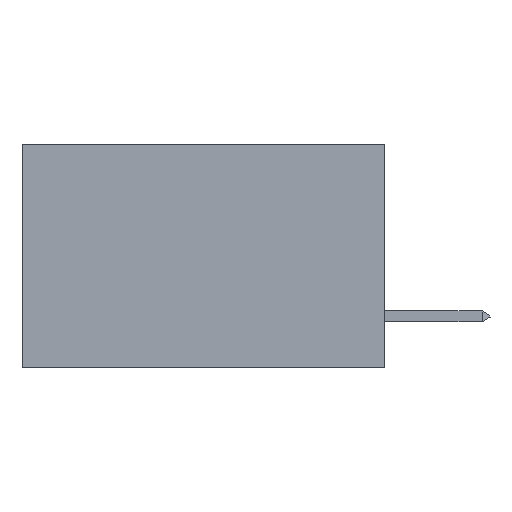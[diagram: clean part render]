
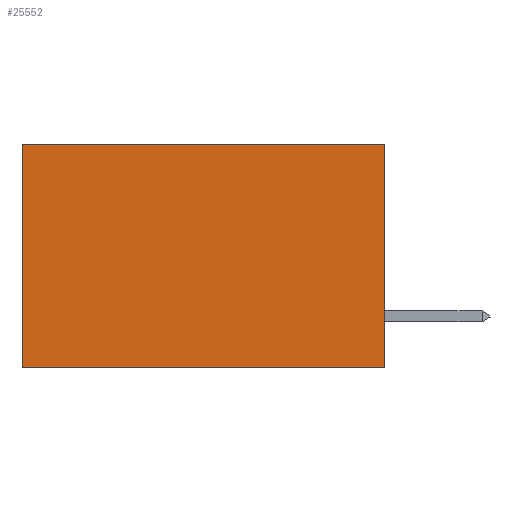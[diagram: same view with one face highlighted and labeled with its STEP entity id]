
A CAD part, left-side view. The second image highlights one B-rep face of the part: STEP entity #25552.
In plain terms, the highlighted planar face has unit normal (-1, 0, 0).
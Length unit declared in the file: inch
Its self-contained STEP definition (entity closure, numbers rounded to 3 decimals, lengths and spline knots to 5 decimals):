
#113 = EDGE_LOOP ( 'NONE', ( #18120, #8792, #2222, #19200 ) ) ;
#640 = DIRECTION ( 'NONE',  ( 0., 1., 0. ) ) ;
#1634 = VERTEX_POINT ( 'NONE', #12951 ) ;
#2222 = ORIENTED_EDGE ( 'NONE', *, *, #30428, .F. ) ;
#2575 = DIRECTION ( 'NONE',  ( 0., 0., -1. ) ) ;
#3344 = DIRECTION ( 'NONE',  ( 0., 0., -1. ) ) ;
#3620 = CARTESIAN_POINT ( 'NONE',  ( 0.2875, 0., -0.37 ) ) ;
#7477 = FACE_OUTER_BOUND ( 'NONE', #113, .T. ) ;
#8740 = LINE ( 'NONE', #19917, #25489 ) ;
#8792 = ORIENTED_EDGE ( 'NONE', *, *, #28315, .F. ) ;
#12466 = VERTEX_POINT ( 'NONE', #20766 ) ;
#12951 = CARTESIAN_POINT ( 'NONE',  ( 0.2875, 0., 0. ) ) ;
#13256 = VECTOR ( 'NONE', #23336, 39.37008 ) ;
#13271 = CARTESIAN_POINT ( 'NONE',  ( 0.2875, 0., 0. ) ) ;
#15188 = VECTOR ( 'NONE', #3344, 39.37008 ) ;
#17224 = DIRECTION ( 'NONE',  ( 0., 0., -1. ) ) ;
#18120 = ORIENTED_EDGE ( 'NONE', *, *, #25185, .T. ) ;
#18304 = CARTESIAN_POINT ( 'NONE',  ( 0.2875, 0.6, -0.37 ) ) ;
#18624 = PLANE ( 'NONE',  #26337 ) ;
#18912 = LINE ( 'NONE', #13271, #15188 ) ;
#19200 = ORIENTED_EDGE ( 'NONE', *, *, #26261, .T. ) ;
#19917 = CARTESIAN_POINT ( 'NONE',  ( 0.2875, 0.6, 0. ) ) ;
#20766 = CARTESIAN_POINT ( 'NONE',  ( 0.2875, 0., -0.37 ) ) ;
#23336 = DIRECTION ( 'NONE',  ( 0., 1., 0. ) ) ;
#23638 = CARTESIAN_POINT ( 'NONE',  ( 0.2875, 0., 0. ) ) ;
#23996 = VERTEX_POINT ( 'NONE', #31749 ) ;
#24476 = VECTOR ( 'NONE', #640, 39.37008 ) ;
#25185 = EDGE_CURVE ( 'NONE', #23996, #28552, #8740, .T. ) ;
#25489 = VECTOR ( 'NONE', #17224, 39.37008 ) ;
#25552 = ADVANCED_FACE ( 'NONE', ( #7477 ), #18624, .F. ) ;
#26261 = EDGE_CURVE ( 'NONE', #1634, #23996, #29100, .T. ) ;
#26337 = AXIS2_PLACEMENT_3D ( 'NONE', #23638, #34285, #2575 ) ;
#28315 = EDGE_CURVE ( 'NONE', #12466, #28552, #29475, .T. ) ;
#28552 = VERTEX_POINT ( 'NONE', #18304 ) ;
#29100 = LINE ( 'NONE', #34126, #13256 ) ;
#29475 = LINE ( 'NONE', #3620, #24476 ) ;
#30428 = EDGE_CURVE ( 'NONE', #1634, #12466, #18912, .T. ) ;
#31749 = CARTESIAN_POINT ( 'NONE',  ( 0.2875, 0.6, 0. ) ) ;
#34126 = CARTESIAN_POINT ( 'NONE',  ( 0.2875, 0., 0. ) ) ;
#34285 = DIRECTION ( 'NONE',  ( 1., 0., 0. ) ) ;
